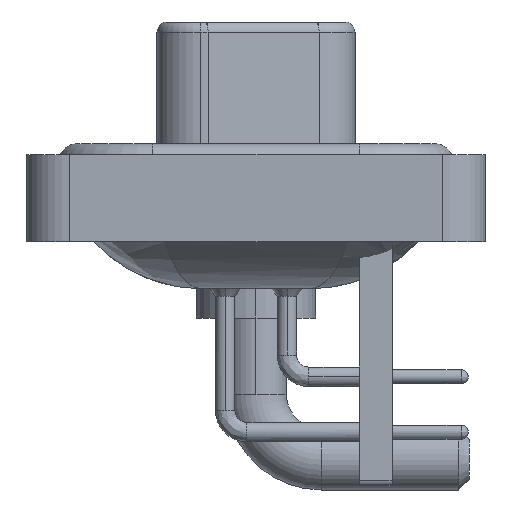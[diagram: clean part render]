
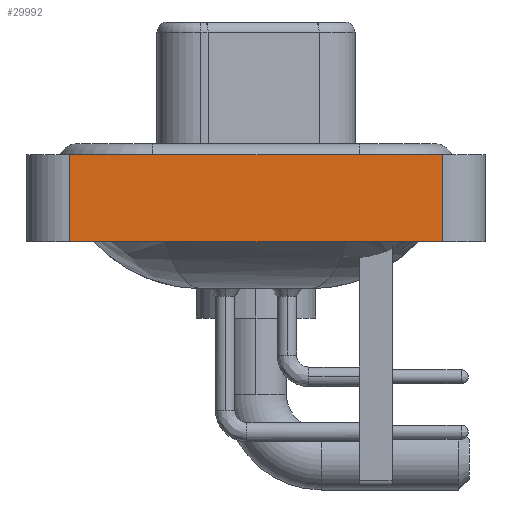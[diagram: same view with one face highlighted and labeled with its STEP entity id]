
A CAD part, left-side view. The second image highlights one B-rep face of the part: STEP entity #29992.
In plain terms, the highlighted planar face has unit normal (-1, 0, 0).
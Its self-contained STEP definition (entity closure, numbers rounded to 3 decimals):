
#281 = VECTOR ( 'NONE', #12544, 1000. ) ;
#522 = EDGE_CURVE ( 'NONE', #28295, #10478, #24051, .T. ) ;
#563 = EDGE_CURVE ( 'NONE', #16014, #10478, #5343, .T. ) ;
#3022 = CARTESIAN_POINT ( 'NONE',  ( -7.35, -8.55, 0.4 ) ) ;
#4057 = FACE_OUTER_BOUND ( 'NONE', #11802, .T. ) ;
#4220 = DIRECTION ( 'NONE',  ( 0., 0., 1. ) ) ;
#4618 = EDGE_CURVE ( 'NONE', #8030, #16014, #23534, .T. ) ;
#5343 = LINE ( 'NONE', #21902, #281 ) ;
#6975 = CARTESIAN_POINT ( 'NONE',  ( -7.35, -8.55, -3.6 ) ) ;
#8030 = VERTEX_POINT ( 'NONE', #26409 ) ;
#8036 = ORIENTED_EDGE ( 'NONE', *, *, #4618, .T. ) ;
#10478 = VERTEX_POINT ( 'NONE', #30106 ) ;
#11254 = CARTESIAN_POINT ( 'NONE',  ( -7.35, -8.55, -3.6 ) ) ;
#11276 = DIRECTION ( 'NONE',  ( -1., 0., 0. ) ) ;
#11802 = EDGE_LOOP ( 'NONE', ( #14982, #17268, #18432, #8036 ) ) ;
#12544 = DIRECTION ( 'NONE',  ( 0., 0., 1. ) ) ;
#14838 = DIRECTION ( 'NONE',  ( 0., -1., 0. ) ) ;
#14982 = ORIENTED_EDGE ( 'NONE', *, *, #563, .T. ) ;
#16014 = VERTEX_POINT ( 'NONE', #11254 ) ;
#16700 = LINE ( 'NONE', #19135, #25333 ) ;
#17268 = ORIENTED_EDGE ( 'NONE', *, *, #522, .F. ) ;
#18432 = ORIENTED_EDGE ( 'NONE', *, *, #28106, .F. ) ;
#19135 = CARTESIAN_POINT ( 'NONE',  ( -7.35, 8.55, -3.6 ) ) ;
#20319 = PLANE ( 'NONE',  #20410 ) ;
#20410 = AXIS2_PLACEMENT_3D ( 'NONE', #25395, #11276, #4220 ) ;
#21902 = CARTESIAN_POINT ( 'NONE',  ( -7.35, -8.55, -3.6 ) ) ;
#22051 = CARTESIAN_POINT ( 'NONE',  ( -7.35, 8.55, 0.4 ) ) ;
#23534 = LINE ( 'NONE', #6975, #27533 ) ;
#24051 = LINE ( 'NONE', #3022, #25285 ) ;
#25285 = VECTOR ( 'NONE', #14838, 1000. ) ;
#25333 = VECTOR ( 'NONE', #28219, 1000. ) ;
#25395 = CARTESIAN_POINT ( 'NONE',  ( -7.35, -8.55, -3.6 ) ) ;
#26409 = CARTESIAN_POINT ( 'NONE',  ( -7.35, 8.55, -3.6 ) ) ;
#27533 = VECTOR ( 'NONE', #30295, 1000. ) ;
#28106 = EDGE_CURVE ( 'NONE', #8030, #28295, #16700, .T. ) ;
#28219 = DIRECTION ( 'NONE',  ( 0., 0., 1. ) ) ;
#28295 = VERTEX_POINT ( 'NONE', #22051 ) ;
#29992 = ADVANCED_FACE ( 'NONE', ( #4057 ), #20319, .T. ) ;
#30106 = CARTESIAN_POINT ( 'NONE',  ( -7.35, -8.55, 0.4 ) ) ;
#30295 = DIRECTION ( 'NONE',  ( 0., -1., 0. ) ) ;
